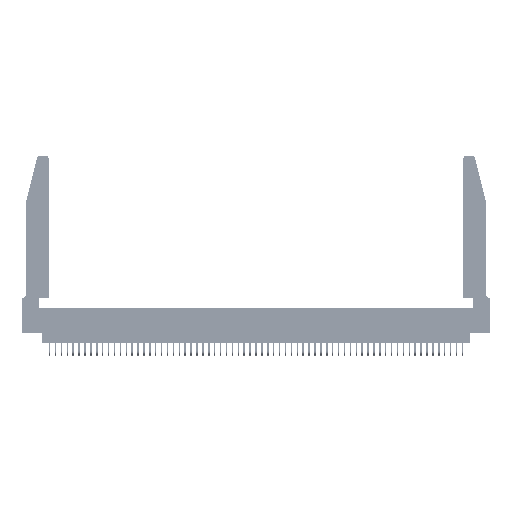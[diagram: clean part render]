
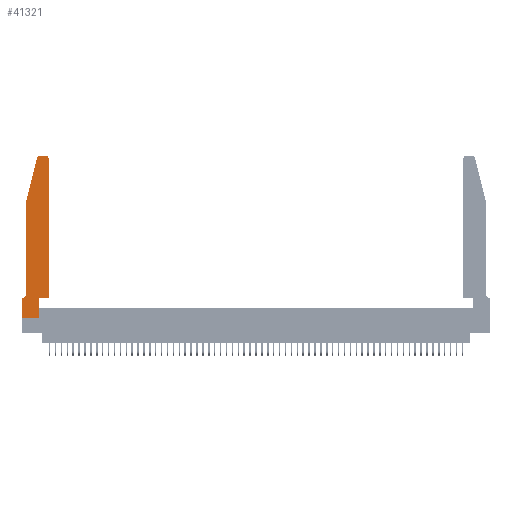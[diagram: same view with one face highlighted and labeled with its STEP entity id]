
A CAD part, top view. The second image highlights one B-rep face of the part: STEP entity #41321.
In plain terms, the highlighted planar face has unit normal (0, 0, 1).
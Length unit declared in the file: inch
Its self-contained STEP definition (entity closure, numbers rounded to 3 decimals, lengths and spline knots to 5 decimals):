
#298 = EDGE_CURVE ( 'NONE', #24753, #16500, #45923, .T. ) ;
#1552 = LINE ( 'NONE', #41253, #53761 ) ;
#1970 = DIRECTION ( 'NONE',  ( -0.239, -0.971, 0. ) ) ;
#2409 = CARTESIAN_POINT ( 'NONE',  ( 0., 0.35, 0.37 ) ) ;
#3987 = ORIENTED_EDGE ( 'NONE', *, *, #18097, .T. ) ;
#5177 = VECTOR ( 'NONE', #57274, 39.37008 ) ;
#5362 = DIRECTION ( 'NONE',  ( 0., 0., -1. ) ) ;
#6177 = CARTESIAN_POINT ( 'NONE',  ( 0.4505, 0.35, 0.37 ) ) ;
#6218 = VECTOR ( 'NONE', #15853, 39.37008 ) ;
#6992 = VERTEX_POINT ( 'NONE', #16016 ) ;
#7100 = FACE_OUTER_BOUND ( 'NONE', #40406, .T. ) ;
#7152 = CIRCLE ( 'NONE', #9940, 0.07 ) ;
#8066 = DIRECTION ( 'NONE',  ( -1., 0., 0. ) ) ;
#8287 = PLANE ( 'NONE',  #38332 ) ;
#8326 = LINE ( 'NONE', #56073, #6218 ) ;
#9462 = DIRECTION ( 'NONE',  ( 1., 0., 0. ) ) ;
#9940 = AXIS2_PLACEMENT_3D ( 'NONE', #27858, #5362, #38118 ) ;
#10014 = CARTESIAN_POINT ( 'NONE',  ( 0., 0., 0.37 ) ) ;
#10549 = EDGE_CURVE ( 'NONE', #27131, #30545, #8326, .T. ) ;
#11847 = VECTOR ( 'NONE', #51338, 39.37008 ) ;
#13058 = EDGE_CURVE ( 'NONE', #14638, #44728, #41195, .T. ) ;
#14194 = CARTESIAN_POINT ( 'NONE',  ( 0.4205, 2.72, 0.37 ) ) ;
#14581 = DIRECTION ( 'NONE',  ( 0., 0., 1. ) ) ;
#14638 = VERTEX_POINT ( 'NONE', #19976 ) ;
#14768 = CIRCLE ( 'NONE', #33169, 0.03 ) ;
#15673 = VECTOR ( 'NONE', #18816, 39.37008 ) ;
#15853 = DIRECTION ( 'NONE',  ( 1., 0., 0. ) ) ;
#16016 = CARTESIAN_POINT ( 'NONE',  ( 0.0055, 0.35, 0.37 ) ) ;
#16500 = VERTEX_POINT ( 'NONE', #51715 ) ;
#17993 = VERTEX_POINT ( 'NONE', #48231 ) ;
#18097 = EDGE_CURVE ( 'NONE', #21071, #17993, #41166, .T. ) ;
#18256 = DIRECTION ( 'NONE',  ( 1., 0., 0. ) ) ;
#18816 = DIRECTION ( 'NONE',  ( 0., -1., 0. ) ) ;
#19323 = LINE ( 'NONE', #57543, #36994 ) ;
#19784 = LINE ( 'NONE', #33904, #36710 ) ;
#19976 = CARTESIAN_POINT ( 'NONE',  ( 0.25487, 2.72718, 0.37 ) ) ;
#20014 = EDGE_CURVE ( 'NONE', #16500, #21071, #14768, .T. ) ;
#20533 = ORIENTED_EDGE ( 'NONE', *, *, #13058, .T. ) ;
#21071 = VERTEX_POINT ( 'NONE', #30860 ) ;
#21256 = ORIENTED_EDGE ( 'NONE', *, *, #26554, .T. ) ;
#21365 = CARTESIAN_POINT ( 'NONE',  ( 0.0755, 0.42, 0.37 ) ) ;
#21706 = CARTESIAN_POINT ( 'NONE',  ( 0.2865, 0., 0.37 ) ) ;
#21843 = ORIENTED_EDGE ( 'NONE', *, *, #52733, .T. ) ;
#21967 = VERTEX_POINT ( 'NONE', #54964 ) ;
#23826 = EDGE_CURVE ( 'NONE', #6992, #47314, #19323, .T. ) ;
#24624 = EDGE_CURVE ( 'NONE', #44728, #35254, #39710, .T. ) ;
#24753 = VERTEX_POINT ( 'NONE', #46984 ) ;
#26554 = EDGE_CURVE ( 'NONE', #21967, #24753, #57041, .T. ) ;
#26812 = ORIENTED_EDGE ( 'NONE', *, *, #24624, .T. ) ;
#27131 = VERTEX_POINT ( 'NONE', #10014 ) ;
#27858 = CARTESIAN_POINT ( 'NONE',  ( 0.0055, 0.42, 0.37 ) ) ;
#29052 = ORIENTED_EDGE ( 'NONE', *, *, #10549, .T. ) ;
#30545 = VERTEX_POINT ( 'NONE', #21706 ) ;
#30860 = CARTESIAN_POINT ( 'NONE',  ( 0.4205, 2.75, 0.37 ) ) ;
#31281 = ORIENTED_EDGE ( 'NONE', *, *, #20014, .T. ) ;
#32032 = DIRECTION ( 'NONE',  ( 0., 1., 0. ) ) ;
#33169 = AXIS2_PLACEMENT_3D ( 'NONE', #14194, #14581, #9462 ) ;
#33904 = CARTESIAN_POINT ( 'NONE',  ( 0., 0., 0.37 ) ) ;
#33936 = ORIENTED_EDGE ( 'NONE', *, *, #23826, .T. ) ;
#34177 = VECTOR ( 'NONE', #1970, 39.37008 ) ;
#34508 = CARTESIAN_POINT ( 'NONE',  ( 0.4505, 0.35, 0.37 ) ) ;
#35254 = VERTEX_POINT ( 'NONE', #21365 ) ;
#35519 = EDGE_CURVE ( 'NONE', #30545, #21967, #1552, .T. ) ;
#35534 = DIRECTION ( 'NONE',  ( 1., 0., 0. ) ) ;
#36235 = DIRECTION ( 'NONE',  ( 0., 0., 1. ) ) ;
#36364 = CIRCLE ( 'NONE', #49866, 0.03 ) ;
#36710 = VECTOR ( 'NONE', #51987, 39.37008 ) ;
#36816 = CARTESIAN_POINT ( 'NONE',  ( 0.284, 2.72, 0.37 ) ) ;
#36994 = VECTOR ( 'NONE', #8066, 39.37008 ) ;
#37700 = CARTESIAN_POINT ( 'NONE',  ( 0.0755, 2., 0.37 ) ) ;
#38118 = DIRECTION ( 'NONE',  ( -1., 0., 0. ) ) ;
#38332 = AXIS2_PLACEMENT_3D ( 'NONE', #57367, #39855, #35534 ) ;
#39033 = DIRECTION ( 'NONE',  ( 0., 1., 0. ) ) ;
#39710 = LINE ( 'NONE', #45823, #15673 ) ;
#39855 = DIRECTION ( 'NONE',  ( 0., 0., 1. ) ) ;
#40406 = EDGE_LOOP ( 'NONE', ( #3987, #45331, #20533, #26812, #41790, #33936, #21843, #29052, #46548, #21256, #50308, #31281 ) ) ;
#41005 = EDGE_CURVE ( 'NONE', #35254, #6992, #7152, .T. ) ;
#41166 = LINE ( 'NONE', #47836, #5177 ) ;
#41195 = LINE ( 'NONE', #37700, #34177 ) ;
#41253 = CARTESIAN_POINT ( 'NONE',  ( 0.2865, 0.35, 0.37 ) ) ;
#41321 = ADVANCED_FACE ( 'NONE', ( #7100 ), #8287, .T. ) ;
#41790 = ORIENTED_EDGE ( 'NONE', *, *, #41005, .T. ) ;
#44524 = VECTOR ( 'NONE', #39033, 39.37008 ) ;
#44728 = VERTEX_POINT ( 'NONE', #57855 ) ;
#45331 = ORIENTED_EDGE ( 'NONE', *, *, #49116, .T. ) ;
#45823 = CARTESIAN_POINT ( 'NONE',  ( 0.0755, 2., 0.37 ) ) ;
#45923 = LINE ( 'NONE', #34508, #44524 ) ;
#46548 = ORIENTED_EDGE ( 'NONE', *, *, #35519, .T. ) ;
#46984 = CARTESIAN_POINT ( 'NONE',  ( 0.4505, 0.35, 0.37 ) ) ;
#47314 = VERTEX_POINT ( 'NONE', #2409 ) ;
#47836 = CARTESIAN_POINT ( 'NONE',  ( 0.2605, 2.75, 0.37 ) ) ;
#48231 = CARTESIAN_POINT ( 'NONE',  ( 0.284, 2.75, 0.37 ) ) ;
#49116 = EDGE_CURVE ( 'NONE', #17993, #14638, #36364, .T. ) ;
#49866 = AXIS2_PLACEMENT_3D ( 'NONE', #36816, #36235, #18256 ) ;
#50308 = ORIENTED_EDGE ( 'NONE', *, *, #298, .T. ) ;
#51338 = DIRECTION ( 'NONE',  ( 1., 0., 0. ) ) ;
#51715 = CARTESIAN_POINT ( 'NONE',  ( 0.4505, 2.72, 0.37 ) ) ;
#51987 = DIRECTION ( 'NONE',  ( 0., -1., 0. ) ) ;
#52733 = EDGE_CURVE ( 'NONE', #47314, #27131, #19784, .T. ) ;
#53761 = VECTOR ( 'NONE', #32032, 39.37008 ) ;
#54964 = CARTESIAN_POINT ( 'NONE',  ( 0.2865, 0.35, 0.37 ) ) ;
#56073 = CARTESIAN_POINT ( 'NONE',  ( 0., 0., 0.37 ) ) ;
#57041 = LINE ( 'NONE', #6177, #11847 ) ;
#57274 = DIRECTION ( 'NONE',  ( -1., 0., 0. ) ) ;
#57367 = CARTESIAN_POINT ( 'NONE',  ( 0., 0.35, 0.37 ) ) ;
#57543 = CARTESIAN_POINT ( 'NONE',  ( 0.0755, 0.35, 0.37 ) ) ;
#57855 = CARTESIAN_POINT ( 'NONE',  ( 0.0755, 2., 0.37 ) ) ;
